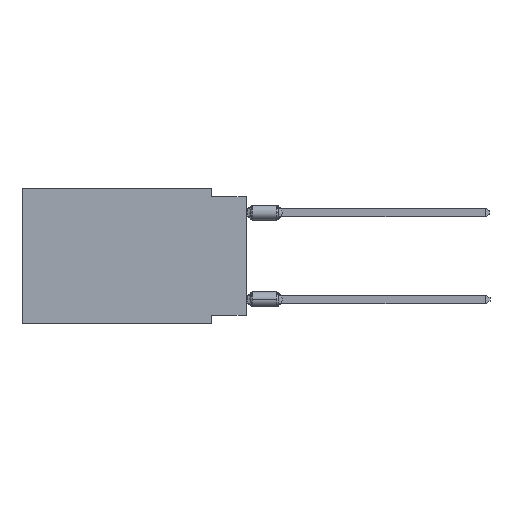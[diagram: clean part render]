
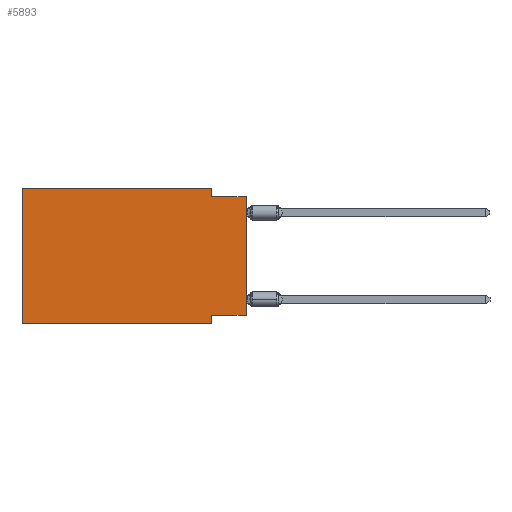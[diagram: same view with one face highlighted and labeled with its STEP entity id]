
A CAD part, left-side view. The second image highlights one B-rep face of the part: STEP entity #5893.
In plain terms, the highlighted planar face has unit normal (-1, 0, 0).
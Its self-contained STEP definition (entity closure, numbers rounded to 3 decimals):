
#733 = EDGE_CURVE ( 'NONE', #28312, #19028, #17689, .T. ) ;
#975 = DIRECTION ( 'NONE',  ( 0., -1., 0. ) ) ;
#1944 = CARTESIAN_POINT ( 'NONE',  ( 0., 0., -9.271 ) ) ;
#2161 = ORIENTED_EDGE ( 'NONE', *, *, #22791, .F. ) ;
#3922 = VECTOR ( 'NONE', #6575, 1000. ) ;
#4336 = VERTEX_POINT ( 'NONE', #29056 ) ;
#4690 = VERTEX_POINT ( 'NONE', #14508 ) ;
#5033 = PLANE ( 'NONE',  #26751 ) ;
#5488 = ORIENTED_EDGE ( 'NONE', *, *, #19088, .F. ) ;
#5642 = CARTESIAN_POINT ( 'NONE',  ( 0., 0., -0.635 ) ) ;
#5893 = ADVANCED_FACE ( 'NONE', ( #7546 ), #5033, .F. ) ;
#6129 = ORIENTED_EDGE ( 'NONE', *, *, #16513, .F. ) ;
#6575 = DIRECTION ( 'NONE',  ( 0., -1., 0. ) ) ;
#7546 = FACE_OUTER_BOUND ( 'NONE', #23450, .T. ) ;
#8329 = LINE ( 'NONE', #10686, #11298 ) ;
#8375 = DIRECTION ( 'NONE',  ( 0., -1., 0. ) ) ;
#8609 = CARTESIAN_POINT ( 'NONE',  ( 0., 16.383, 0. ) ) ;
#8669 = ORIENTED_EDGE ( 'NONE', *, *, #22590, .T. ) ;
#10068 = DIRECTION ( 'NONE',  ( 1., 0., 0. ) ) ;
#10288 = CARTESIAN_POINT ( 'NONE',  ( 0., 16.383, -9.906 ) ) ;
#10686 = CARTESIAN_POINT ( 'NONE',  ( 0., 0., 0. ) ) ;
#10926 = VECTOR ( 'NONE', #30898, 1000. ) ;
#10980 = EDGE_CURVE ( 'NONE', #29057, #4690, #19133, .T. ) ;
#11152 = CARTESIAN_POINT ( 'NONE',  ( 0., 0., -0.635 ) ) ;
#11298 = VECTOR ( 'NONE', #20465, 1000. ) ;
#11467 = ORIENTED_EDGE ( 'NONE', *, *, #14204, .F. ) ;
#11596 = LINE ( 'NONE', #21223, #15346 ) ;
#11751 = ORIENTED_EDGE ( 'NONE', *, *, #733, .T. ) ;
#13106 = CARTESIAN_POINT ( 'NONE',  ( 0., 2.54, -9.906 ) ) ;
#13810 = DIRECTION ( 'NONE',  ( 0., 0., 1. ) ) ;
#14204 = EDGE_CURVE ( 'NONE', #28312, #26590, #16643, .T. ) ;
#14508 = CARTESIAN_POINT ( 'NONE',  ( 0., 2.54, -9.271 ) ) ;
#14799 = CARTESIAN_POINT ( 'NONE',  ( 0., 16.383, 0. ) ) ;
#15050 = ORIENTED_EDGE ( 'NONE', *, *, #17712, .F. ) ;
#15100 = VECTOR ( 'NONE', #975, 1000. ) ;
#15208 = VERTEX_POINT ( 'NONE', #17638 ) ;
#15346 = VECTOR ( 'NONE', #19174, 1000. ) ;
#15978 = VECTOR ( 'NONE', #18515, 1000. ) ;
#16080 = CARTESIAN_POINT ( 'NONE',  ( 0., 2.54, -9.906 ) ) ;
#16513 = EDGE_CURVE ( 'NONE', #15208, #26509, #25525, .T. ) ;
#16643 = LINE ( 'NONE', #19017, #22079 ) ;
#17537 = CARTESIAN_POINT ( 'NONE',  ( 0., 16.383, 0. ) ) ;
#17638 = CARTESIAN_POINT ( 'NONE',  ( 0., 2.54, -0.635 ) ) ;
#17689 = LINE ( 'NONE', #10288, #15100 ) ;
#17712 = EDGE_CURVE ( 'NONE', #26590, #4336, #27009, .T. ) ;
#18515 = DIRECTION ( 'NONE',  ( 0., 1., 0. ) ) ;
#19017 = CARTESIAN_POINT ( 'NONE',  ( 0., 16.383, 0. ) ) ;
#19028 = VERTEX_POINT ( 'NONE', #13106 ) ;
#19088 = EDGE_CURVE ( 'NONE', #4690, #19028, #23638, .T. ) ;
#19133 = LINE ( 'NONE', #1944, #15978 ) ;
#19174 = DIRECTION ( 'NONE',  ( 0., 0., -1. ) ) ;
#19942 = VECTOR ( 'NONE', #8375, 1000. ) ;
#20415 = DIRECTION ( 'NONE',  ( 0., 0., -1. ) ) ;
#20465 = DIRECTION ( 'NONE',  ( 0., 0., 1. ) ) ;
#20596 = ORIENTED_EDGE ( 'NONE', *, *, #10980, .F. ) ;
#21223 = CARTESIAN_POINT ( 'NONE',  ( 0., 2.54, 0. ) ) ;
#22079 = VECTOR ( 'NONE', #13810, 1000. ) ;
#22590 = EDGE_CURVE ( 'NONE', #29057, #26509, #8329, .T. ) ;
#22791 = EDGE_CURVE ( 'NONE', #4336, #15208, #11596, .T. ) ;
#23434 = CARTESIAN_POINT ( 'NONE',  ( 0., 0., -9.271 ) ) ;
#23450 = EDGE_LOOP ( 'NONE', ( #8669, #6129, #2161, #15050, #11467, #11751, #5488, #20596 ) ) ;
#23638 = LINE ( 'NONE', #16080, #10926 ) ;
#25525 = LINE ( 'NONE', #11152, #3922 ) ;
#26403 = CARTESIAN_POINT ( 'NONE',  ( 0., 16.383, -9.906 ) ) ;
#26509 = VERTEX_POINT ( 'NONE', #5642 ) ;
#26590 = VERTEX_POINT ( 'NONE', #8609 ) ;
#26751 = AXIS2_PLACEMENT_3D ( 'NONE', #14799, #10068, #20415 ) ;
#27009 = LINE ( 'NONE', #17537, #19942 ) ;
#28312 = VERTEX_POINT ( 'NONE', #26403 ) ;
#29056 = CARTESIAN_POINT ( 'NONE',  ( 0., 2.54, 0. ) ) ;
#29057 = VERTEX_POINT ( 'NONE', #23434 ) ;
#30898 = DIRECTION ( 'NONE',  ( 0., 0., -1. ) ) ;
